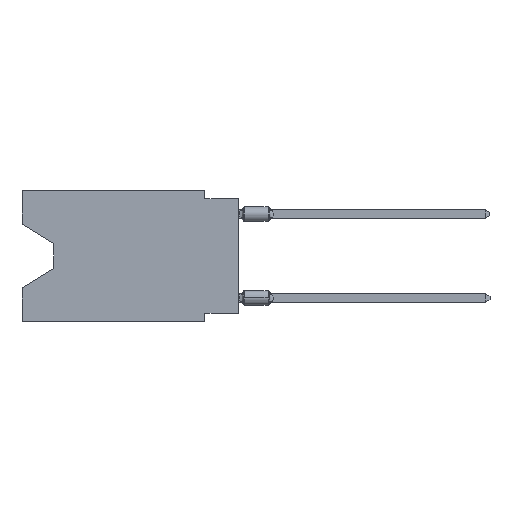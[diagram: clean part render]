
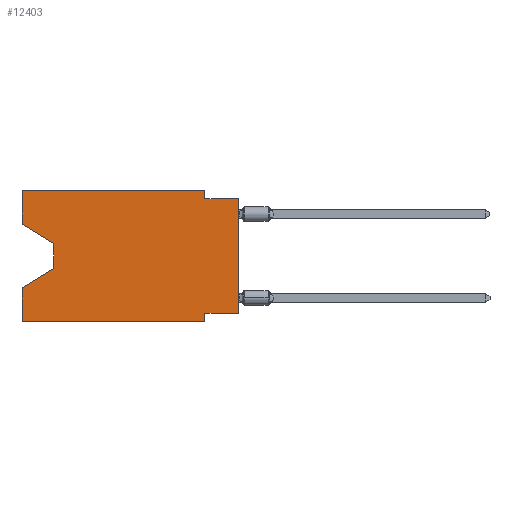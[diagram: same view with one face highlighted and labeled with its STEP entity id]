
A CAD part, left-side view. The second image highlights one B-rep face of the part: STEP entity #12403.
In plain terms, the highlighted planar face has unit normal (-1, 0, 0).
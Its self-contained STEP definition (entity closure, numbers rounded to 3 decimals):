
#7 = VERTEX_POINT ( 'NONE', #11879 ) ;
#16 = ORIENTED_EDGE ( 'NONE', *, *, #5849, .T. ) ;
#69 = DIRECTION ( 'NONE',  ( 0., 0., -1. ) ) ;
#406 = CARTESIAN_POINT ( 'NONE',  ( 0., 2.54, -9.906 ) ) ;
#407 = VECTOR ( 'NONE', #5148, 1000. ) ;
#471 = VECTOR ( 'NONE', #7947, 1000. ) ;
#900 = CARTESIAN_POINT ( 'NONE',  ( 0., 2.54, 0. ) ) ;
#1083 = LINE ( 'NONE', #900, #471 ) ;
#1084 = LINE ( 'NONE', #8421, #17294 ) ;
#1231 = CARTESIAN_POINT ( 'NONE',  ( 0., 0., -0.635 ) ) ;
#1489 = PLANE ( 'NONE',  #12420 ) ;
#1578 = CARTESIAN_POINT ( 'NONE',  ( 0., 16.383, 0. ) ) ;
#1595 = LINE ( 'NONE', #10059, #16955 ) ;
#1634 = LINE ( 'NONE', #15931, #4625 ) ;
#2062 = ORIENTED_EDGE ( 'NONE', *, *, #18483, .F. ) ;
#2713 = CARTESIAN_POINT ( 'NONE',  ( 0., 2.54, 0. ) ) ;
#2964 = VECTOR ( 'NONE', #4079, 1000. ) ;
#3106 = LINE ( 'NONE', #406, #7126 ) ;
#3244 = DIRECTION ( 'NONE',  ( 0., 0., 1. ) ) ;
#3663 = EDGE_CURVE ( 'NONE', #16015, #15372, #7940, .T. ) ;
#4079 = DIRECTION ( 'NONE',  ( 0., 0., 1. ) ) ;
#4202 = CARTESIAN_POINT ( 'NONE',  ( 0., 16.383, -7.36 ) ) ;
#4215 = FACE_OUTER_BOUND ( 'NONE', #9487, .T. ) ;
#4366 = CARTESIAN_POINT ( 'NONE',  ( 0., 16.383, 0. ) ) ;
#4584 = LINE ( 'NONE', #12881, #13710 ) ;
#4625 = VECTOR ( 'NONE', #3244, 1000. ) ;
#5148 = DIRECTION ( 'NONE',  ( 0., -1., 0. ) ) ;
#5370 = DIRECTION ( 'NONE',  ( 0., -1., 0. ) ) ;
#5475 = VERTEX_POINT ( 'NONE', #6127 ) ;
#5849 = EDGE_CURVE ( 'NONE', #9464, #15929, #1595, .T. ) ;
#5881 = VERTEX_POINT ( 'NONE', #7241 ) ;
#6127 = CARTESIAN_POINT ( 'NONE',  ( 0., 2.54, -0.635 ) ) ;
#7126 = VECTOR ( 'NONE', #12966, 1000. ) ;
#7241 = CARTESIAN_POINT ( 'NONE',  ( 0., 0., -9.271 ) ) ;
#7335 = DIRECTION ( 'NONE',  ( 0., 0., -1. ) ) ;
#7672 = CARTESIAN_POINT ( 'NONE',  ( 0., 16.383, -9.906 ) ) ;
#7857 = CARTESIAN_POINT ( 'NONE',  ( 0., 2.54, -9.271 ) ) ;
#7940 = LINE ( 'NONE', #8316, #2964 ) ;
#7947 = DIRECTION ( 'NONE',  ( 0., 0., -1. ) ) ;
#8074 = LINE ( 'NONE', #18397, #407 ) ;
#8230 = DIRECTION ( 'NONE',  ( 0., 0., 1. ) ) ;
#8316 = CARTESIAN_POINT ( 'NONE',  ( 0., 16.383, 0. ) ) ;
#8400 = ORIENTED_EDGE ( 'NONE', *, *, #11145, .T. ) ;
#8421 = CARTESIAN_POINT ( 'NONE',  ( 0., 16.383, -2.546 ) ) ;
#8427 = LINE ( 'NONE', #8514, #11330 ) ;
#8505 = LINE ( 'NONE', #16971, #15504 ) ;
#8514 = CARTESIAN_POINT ( 'NONE',  ( 0., 0., 0. ) ) ;
#8595 = ORIENTED_EDGE ( 'NONE', *, *, #9311, .T. ) ;
#8880 = CARTESIAN_POINT ( 'NONE',  ( 0., 13.97, -5.893 ) ) ;
#8973 = EDGE_CURVE ( 'NONE', #10673, #13277, #3106, .T. ) ;
#9311 = EDGE_CURVE ( 'NONE', #5881, #11153, #8427, .T. ) ;
#9464 = VERTEX_POINT ( 'NONE', #16126 ) ;
#9487 = EDGE_LOOP ( 'NONE', ( #15300, #16, #15273, #9741, #8400, #14128, #13837, #8595, #2062, #14579, #16410, #12833 ) ) ;
#9741 = ORIENTED_EDGE ( 'NONE', *, *, #3663, .F. ) ;
#10059 = CARTESIAN_POINT ( 'NONE',  ( 0., 13.97, -4.013 ) ) ;
#10325 = DIRECTION ( 'NONE',  ( 0., 0.855, -0.519 ) ) ;
#10673 = VERTEX_POINT ( 'NONE', #7857 ) ;
#11131 = DIRECTION ( 'NONE',  ( 0., -0.855, -0.519 ) ) ;
#11145 = EDGE_CURVE ( 'NONE', #16015, #13277, #18154, .T. ) ;
#11153 = VERTEX_POINT ( 'NONE', #1231 ) ;
#11330 = VECTOR ( 'NONE', #8230, 1000. ) ;
#11342 = CARTESIAN_POINT ( 'NONE',  ( 0., 16.383, 0. ) ) ;
#11879 = CARTESIAN_POINT ( 'NONE',  ( 0., 16.383, -2.546 ) ) ;
#12074 = VECTOR ( 'NONE', #15754, 1000. ) ;
#12403 = ADVANCED_FACE ( 'NONE', ( #4215 ), #1489, .F. ) ;
#12420 = AXIS2_PLACEMENT_3D ( 'NONE', #1578, #12771, #69 ) ;
#12771 = DIRECTION ( 'NONE',  ( 1., 0., 0. ) ) ;
#12825 = EDGE_CURVE ( 'NONE', #7, #15437, #1634, .T. ) ;
#12833 = ORIENTED_EDGE ( 'NONE', *, *, #12825, .F. ) ;
#12881 = CARTESIAN_POINT ( 'NONE',  ( 0., 13.97, -5.893 ) ) ;
#12966 = DIRECTION ( 'NONE',  ( 0., 0., -1. ) ) ;
#13277 = VERTEX_POINT ( 'NONE', #14597 ) ;
#13710 = VECTOR ( 'NONE', #10325, 1000. ) ;
#13837 = ORIENTED_EDGE ( 'NONE', *, *, #14490, .F. ) ;
#13934 = CARTESIAN_POINT ( 'NONE',  ( 0., 16.383, -9.906 ) ) ;
#14063 = VERTEX_POINT ( 'NONE', #2713 ) ;
#14128 = ORIENTED_EDGE ( 'NONE', *, *, #8973, .F. ) ;
#14333 = EDGE_CURVE ( 'NONE', #14063, #5475, #1083, .T. ) ;
#14490 = EDGE_CURVE ( 'NONE', #5881, #10673, #8505, .T. ) ;
#14579 = ORIENTED_EDGE ( 'NONE', *, *, #14333, .F. ) ;
#14597 = CARTESIAN_POINT ( 'NONE',  ( 0., 2.54, -9.906 ) ) ;
#14927 = EDGE_CURVE ( 'NONE', #15929, #15372, #4584, .T. ) ;
#15273 = ORIENTED_EDGE ( 'NONE', *, *, #14927, .T. ) ;
#15300 = ORIENTED_EDGE ( 'NONE', *, *, #16170, .T. ) ;
#15372 = VERTEX_POINT ( 'NONE', #4202 ) ;
#15437 = VERTEX_POINT ( 'NONE', #11342 ) ;
#15504 = VECTOR ( 'NONE', #17068, 1000. ) ;
#15754 = DIRECTION ( 'NONE',  ( 0., -1., 0. ) ) ;
#15764 = VECTOR ( 'NONE', #5370, 1000. ) ;
#15849 = LINE ( 'NONE', #4366, #12074 ) ;
#15929 = VERTEX_POINT ( 'NONE', #8880 ) ;
#15931 = CARTESIAN_POINT ( 'NONE',  ( 0., 16.383, 0. ) ) ;
#16015 = VERTEX_POINT ( 'NONE', #7672 ) ;
#16126 = CARTESIAN_POINT ( 'NONE',  ( 0., 13.97, -4.013 ) ) ;
#16170 = EDGE_CURVE ( 'NONE', #7, #9464, #1084, .T. ) ;
#16235 = EDGE_CURVE ( 'NONE', #15437, #14063, #15849, .T. ) ;
#16410 = ORIENTED_EDGE ( 'NONE', *, *, #16235, .F. ) ;
#16955 = VECTOR ( 'NONE', #7335, 1000. ) ;
#16971 = CARTESIAN_POINT ( 'NONE',  ( 0., 0., -9.271 ) ) ;
#17068 = DIRECTION ( 'NONE',  ( 0., 1., 0. ) ) ;
#17294 = VECTOR ( 'NONE', #11131, 1000. ) ;
#18154 = LINE ( 'NONE', #13934, #15764 ) ;
#18397 = CARTESIAN_POINT ( 'NONE',  ( 0., 0., -0.635 ) ) ;
#18483 = EDGE_CURVE ( 'NONE', #5475, #11153, #8074, .T. ) ;
